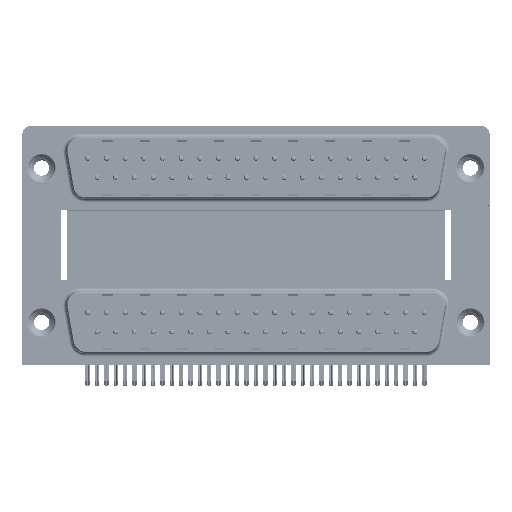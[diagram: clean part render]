
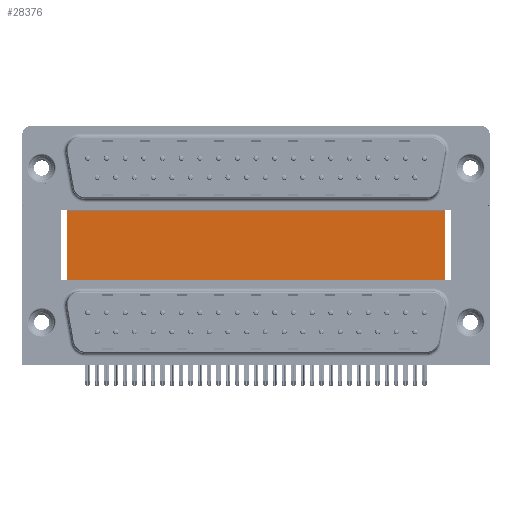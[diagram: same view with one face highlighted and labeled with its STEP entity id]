
A CAD part, top view. The second image highlights one B-rep face of the part: STEP entity #28376.
In plain terms, the highlighted planar face has unit normal (0, 0, 1).
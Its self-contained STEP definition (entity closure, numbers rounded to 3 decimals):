
#240 = VERTEX_POINT ( 'NONE', #32245 ) ;
#1365 = EDGE_CURVE ( 'NONE', #240, #30688, #3830, .T. ) ;
#1498 = LINE ( 'NONE', #22234, #48979 ) ;
#3830 = LINE ( 'NONE', #4359, #16449 ) ;
#4290 = CARTESIAN_POINT ( 'NONE',  ( 3.79, 16.585, -12. ) ) ;
#4359 = CARTESIAN_POINT ( 'NONE',  ( 3.79, -3.735, -12. ) ) ;
#7833 = DIRECTION ( 'NONE',  ( 0., -1., 0. ) ) ;
#8611 = DIRECTION ( 'NONE',  ( 1., 0., 0. ) ) ;
#8681 = DIRECTION ( 'NONE',  ( 1., 0., 0. ) ) ;
#8795 = VERTEX_POINT ( 'NONE', #50703 ) ;
#10002 = AXIS2_PLACEMENT_3D ( 'NONE', #27565, #43974, #28092 ) ;
#10680 = CARTESIAN_POINT ( 'NONE',  ( 59.71, -3.735, -12. ) ) ;
#11142 = FACE_OUTER_BOUND ( 'NONE', #16158, .T. ) ;
#16158 = EDGE_LOOP ( 'NONE', ( #50328, #44700, #41672, #25463 ) ) ;
#16449 = VECTOR ( 'NONE', #8681, 1000. ) ;
#21161 = DIRECTION ( 'NONE',  ( 0., -1., 0. ) ) ;
#22234 = CARTESIAN_POINT ( 'NONE',  ( 59.71, 16.585, -12. ) ) ;
#25463 = ORIENTED_EDGE ( 'NONE', *, *, #43243, .T. ) ;
#27565 = CARTESIAN_POINT ( 'NONE',  ( 3.79, 16.585, -12. ) ) ;
#28092 = DIRECTION ( 'NONE',  ( -1., 0., 0. ) ) ;
#28376 = ADVANCED_FACE ( 'NONE', ( #11142 ), #32108, .F. ) ;
#30688 = VERTEX_POINT ( 'NONE', #10680 ) ;
#32108 = PLANE ( 'NONE',  #10002 ) ;
#32245 = CARTESIAN_POINT ( 'NONE',  ( 3.79, -3.735, -12. ) ) ;
#32401 = VERTEX_POINT ( 'NONE', #36194 ) ;
#36115 = CARTESIAN_POINT ( 'NONE',  ( 3.79, 16.585, -12. ) ) ;
#36194 = CARTESIAN_POINT ( 'NONE',  ( 59.71, 16.585, -12. ) ) ;
#41202 = LINE ( 'NONE', #4290, #41421 ) ;
#41421 = VECTOR ( 'NONE', #8611, 1000. ) ;
#41672 = ORIENTED_EDGE ( 'NONE', *, *, #51498, .F. ) ;
#43243 = EDGE_CURVE ( 'NONE', #8795, #240, #52014, .T. ) ;
#43974 = DIRECTION ( 'NONE',  ( 0., 0., -1. ) ) ;
#44700 = ORIENTED_EDGE ( 'NONE', *, *, #45533, .F. ) ;
#45533 = EDGE_CURVE ( 'NONE', #32401, #30688, #1498, .T. ) ;
#47180 = VECTOR ( 'NONE', #7833, 1000. ) ;
#48979 = VECTOR ( 'NONE', #21161, 1000. ) ;
#50328 = ORIENTED_EDGE ( 'NONE', *, *, #1365, .T. ) ;
#50703 = CARTESIAN_POINT ( 'NONE',  ( 3.79, 16.585, -12. ) ) ;
#51498 = EDGE_CURVE ( 'NONE', #8795, #32401, #41202, .T. ) ;
#52014 = LINE ( 'NONE', #36115, #47180 ) ;
